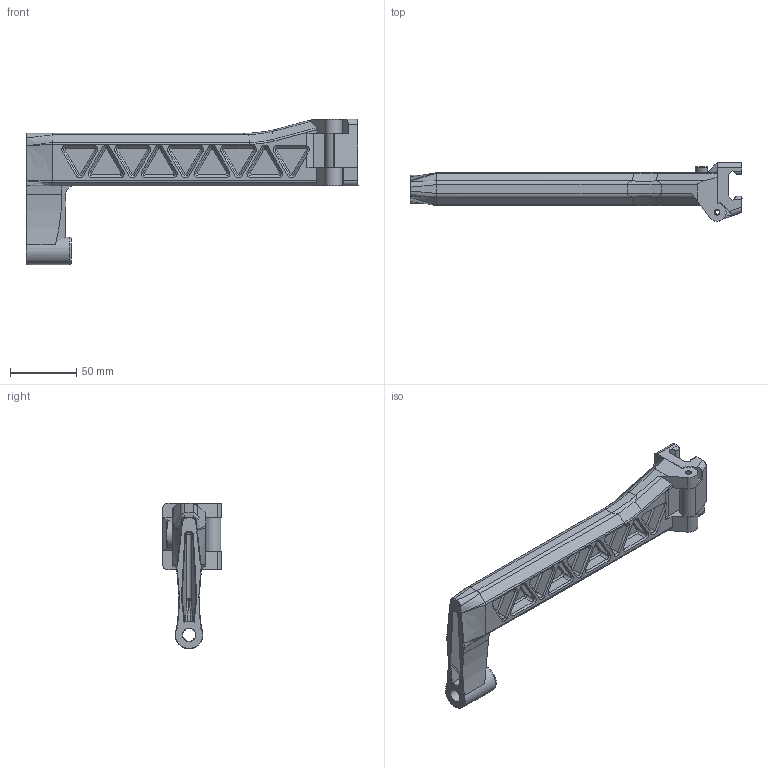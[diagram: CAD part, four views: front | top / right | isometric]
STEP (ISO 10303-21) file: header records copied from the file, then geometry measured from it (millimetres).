
FILE_DESCRIPTION(/* description */ (''),/* implementation_level */ '2;1');
FILE_NAME(/* author */ (''),/* organization */ (''),/* preprocessor_version */ 'ST-DEVELOPER v15.2',/* originating_system */ 'Autodesk Translator Framework v2.0.0.5431',/* authorisation */ '');
FILE_SCHEMA (('AUTOMOTIVE_DESIGN { 1 0 10303 214 3 1 1 }'));
Length unit declared in the file: centimetre
Products named in the file (1): (Unsaved)
Bounding box: 250.99 x 44.3 x 110.03 mm (x, y, z)
Volume: 213056.6 mm3; surface area: 64160.7 mm2
Topology: 3 solids, 3 shells, 587 faces, 1403 edges, 841 vertices
Faces by surface type: plane 300, cone 116, cylinder 112, bspline 54, torus 4, sphere 1
Full cylindrical faces by diameter (mm): 3 x1, 3.6 x2, 4 x1, 9.6 x1, 10 x1, 12.1 x1, 20.5 x1, 21 x1
Entity records: 17591 total; most frequent: CARTESIAN_POINT 4204, ORIENTED_EDGE 2756, DIRECTION 2737, EDGE_CURVE 1378, LINE 929, VECTOR 929, AXIS2_PLACEMENT_3D 904, VERTEX_POINT 835
